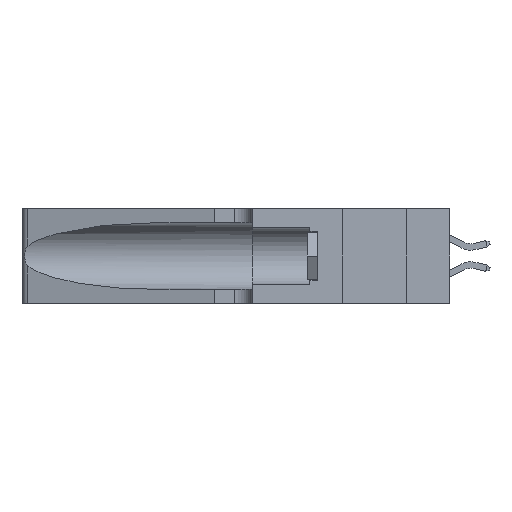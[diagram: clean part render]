
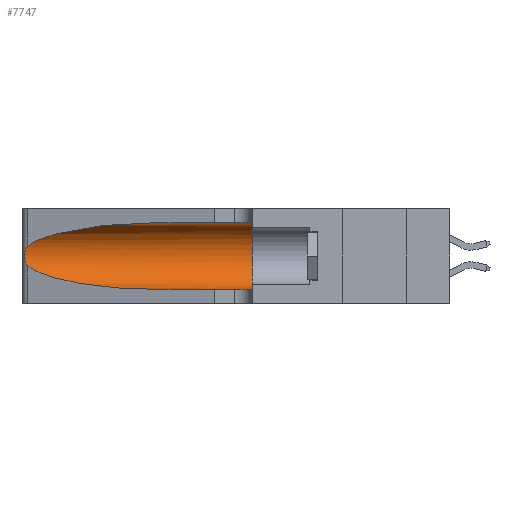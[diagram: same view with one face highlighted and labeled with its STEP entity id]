
A CAD part, left-side view. The second image highlights one B-rep face of the part: STEP entity #7747.
In plain terms, the highlighted cylindrical face has radius 3.308 mm (diameter 6.617 mm), a partial arc.
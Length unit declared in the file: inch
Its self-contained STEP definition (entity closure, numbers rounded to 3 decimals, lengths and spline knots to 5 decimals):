
#30 = CARTESIAN_POINT ( 'NONE',  ( 0.26017, 1.23833, 0.17102 ) ) ;
#671 = CARTESIAN_POINT ( 'NONE',  ( 0.1305, 0.35, 0.05475 ) ) ;
#1017 = EDGE_CURVE ( 'NONE', #13923, #11739, #7935, .T. ) ;
#1211 = CARTESIAN_POINT ( 'NONE',  ( 0.1305, 0.35, 0.31525 ) ) ;
#1793 = CARTESIAN_POINT ( 'NONE',  ( 0.25789, 1.23486, 0.15765 ) ) ;
#1945 = B_SPLINE_CURVE_WITH_KNOTS ( 'NONE', 3,
 ( #15384, #3475, #17036, #6945, #18658, #8681, #20259, #10394, #30, #12070, #1793, #13759, #3551, #15453 ),
 .UNSPECIFIED., .F., .F.,
 ( 4, 2, 2, 2, 2, 2, 4 ),
 ( 0., 0.00027, 0.00053, 0.00107, 0.0016, 0.00187, 0.00214 ),
 .UNSPECIFIED. ) ;
#2214 = EDGE_CURVE ( 'NONE', #11739, #16874, #2476, .T. ) ;
#2233 =( BOUNDED_CURVE ( )  B_SPLINE_CURVE ( 3, ( #11299, #4411, #17861, #12996 ),
 .UNSPECIFIED., .F., .F. ) 
 B_SPLINE_CURVE_WITH_KNOTS ( ( 4, 4 ),
 ( 1.5708, 2.84003 ),
 .UNSPECIFIED. ) 
 CURVE ( )  GEOMETRIC_REPRESENTATION_ITEM ( )  RATIONAL_B_SPLINE_CURVE ( ( 1., 0.87, 0.87, 1. ) ) 
 REPRESENTATION_ITEM ( '' )  );
#2355 =( BOUNDED_CURVE ( )  B_SPLINE_CURVE ( 3, ( #3543, #20253, #5276, #17101 ),
 .UNSPECIFIED., .F., .T. ) 
 B_SPLINE_CURVE_WITH_KNOTS ( ( 4, 4 ),
 ( 3.44316, 4.71239 ),
 .UNSPECIFIED. ) 
 CURVE ( )  GEOMETRIC_REPRESENTATION_ITEM ( )  RATIONAL_B_SPLINE_CURVE ( ( 1., 0.87, 0.87, 1. ) ) 
 REPRESENTATION_ITEM ( '' )  );
#2476 = CIRCLE ( 'NONE', #15909, 0.13025 ) ;
#3250 = DIRECTION ( 'NONE',  ( 0., 0., 1. ) ) ;
#3272 = DIRECTION ( 'NONE',  ( 0., 1., 0. ) ) ;
#3293 = CARTESIAN_POINT ( 'NONE',  ( 0.1305, 0.35, 0.185 ) ) ;
#3475 = CARTESIAN_POINT ( 'NONE',  ( 0.25555, 1.22994, 0.2215 ) ) ;
#3543 = CARTESIAN_POINT ( 'NONE',  ( 0.25487, 1.22718, 0.14631 ) ) ;
#3551 = CARTESIAN_POINT ( 'NONE',  ( 0.25555, 1.22993, 0.14849 ) ) ;
#4208 = CARTESIAN_POINT ( 'NONE',  ( 0.1305, 1.61858, 0.185 ) ) ;
#4411 = CARTESIAN_POINT ( 'NONE',  ( 0.18966, 0.96281, 0.31525 ) ) ;
#5276 = CARTESIAN_POINT ( 'NONE',  ( 0.18966, 0.96281, 0.05475 ) ) ;
#6552 = AXIS2_PLACEMENT_3D ( 'NONE', #4208, #7702, #19351 ) ;
#6945 = CARTESIAN_POINT ( 'NONE',  ( 0.25787, 1.23484, 0.2124 ) ) ;
#7403 = CARTESIAN_POINT ( 'NONE',  ( 0.1305, 1.61858, 0.31525 ) ) ;
#7537 = FACE_OUTER_BOUND ( 'NONE', #17459, .T. ) ;
#7702 = DIRECTION ( 'NONE',  ( 0., -1., 0. ) ) ;
#7727 = CARTESIAN_POINT ( 'NONE',  ( 0.25487, 1.22718, 0.22369 ) ) ;
#7747 = ADVANCED_FACE ( 'NONE', ( #7537 ), #15473, .F. ) ;
#7935 = LINE ( 'NONE', #7403, #11909 ) ;
#8681 = CARTESIAN_POINT ( 'NONE',  ( 0.26018, 1.23835, 0.19895 ) ) ;
#8848 = CARTESIAN_POINT ( 'NONE',  ( 0.1305, 0.72297, 0.31525 ) ) ;
#8923 = CARTESIAN_POINT ( 'NONE',  ( 0.1305, 1.61858, 0.05475 ) ) ;
#9447 = ORIENTED_EDGE ( 'NONE', *, *, #1017, .F. ) ;
#10230 = ORIENTED_EDGE ( 'NONE', *, *, #12921, .T. ) ;
#10394 = CARTESIAN_POINT ( 'NONE',  ( 0.26075, 1.23896, 0.178 ) ) ;
#10628 = DIRECTION ( 'NONE',  ( 0., -1., 0. ) ) ;
#11104 = LINE ( 'NONE', #8923, #15064 ) ;
#11299 = CARTESIAN_POINT ( 'NONE',  ( 0.1305, 0.72297, 0.31525 ) ) ;
#11668 = VERTEX_POINT ( 'NONE', #16318 ) ;
#11739 = VERTEX_POINT ( 'NONE', #1211 ) ;
#11909 = VECTOR ( 'NONE', #20676, 39.37008 ) ;
#11933 = EDGE_CURVE ( 'NONE', #18288, #16874, #11104, .T. ) ;
#12070 = CARTESIAN_POINT ( 'NONE',  ( 0.25856, 1.23593, 0.16098 ) ) ;
#12536 = EDGE_CURVE ( 'NONE', #11668, #18288, #2355, .T. ) ;
#12896 = CARTESIAN_POINT ( 'NONE',  ( 0.1305, 0.72297, 0.05475 ) ) ;
#12921 = EDGE_CURVE ( 'NONE', #13923, #13490, #2233, .T. ) ;
#12996 = CARTESIAN_POINT ( 'NONE',  ( 0.25487, 1.22718, 0.22369 ) ) ;
#13426 = ORIENTED_EDGE ( 'NONE', *, *, #19111, .T. ) ;
#13490 = VERTEX_POINT ( 'NONE', #7727 ) ;
#13759 = CARTESIAN_POINT ( 'NONE',  ( 0.25639, 1.23186, 0.15144 ) ) ;
#13923 = VERTEX_POINT ( 'NONE', #8848 ) ;
#15064 = VECTOR ( 'NONE', #10628, 39.37008 ) ;
#15384 = CARTESIAN_POINT ( 'NONE',  ( 0.25487, 1.22718, 0.22369 ) ) ;
#15453 = CARTESIAN_POINT ( 'NONE',  ( 0.25487, 1.22718, 0.14631 ) ) ;
#15473 = CYLINDRICAL_SURFACE ( 'NONE', #6552, 0.13025 ) ;
#15909 = AXIS2_PLACEMENT_3D ( 'NONE', #3293, #3272, #3250 ) ;
#16188 = ORIENTED_EDGE ( 'NONE', *, *, #2214, .F. ) ;
#16318 = CARTESIAN_POINT ( 'NONE',  ( 0.25487, 1.22718, 0.14631 ) ) ;
#16324 = ORIENTED_EDGE ( 'NONE', *, *, #11933, .T. ) ;
#16874 = VERTEX_POINT ( 'NONE', #671 ) ;
#17036 = CARTESIAN_POINT ( 'NONE',  ( 0.25639, 1.23184, 0.21858 ) ) ;
#17101 = CARTESIAN_POINT ( 'NONE',  ( 0.1305, 0.72297, 0.05475 ) ) ;
#17459 = EDGE_LOOP ( 'NONE', ( #10230, #13426, #19748, #16324, #16188, #9447 ) ) ;
#17861 = CARTESIAN_POINT ( 'NONE',  ( 0.2373, 1.15595, 0.28018 ) ) ;
#18288 = VERTEX_POINT ( 'NONE', #12896 ) ;
#18658 = CARTESIAN_POINT ( 'NONE',  ( 0.25854, 1.2359, 0.20912 ) ) ;
#19111 = EDGE_CURVE ( 'NONE', #13490, #11668, #1945, .T. ) ;
#19351 = DIRECTION ( 'NONE',  ( 0., 0., -1. ) ) ;
#19748 = ORIENTED_EDGE ( 'NONE', *, *, #12536, .T. ) ;
#20253 = CARTESIAN_POINT ( 'NONE',  ( 0.2373, 1.15595, 0.08982 ) ) ;
#20259 = CARTESIAN_POINT ( 'NONE',  ( 0.26075, 1.23896, 0.19203 ) ) ;
#20676 = DIRECTION ( 'NONE',  ( 0., -1., 0. ) ) ;
